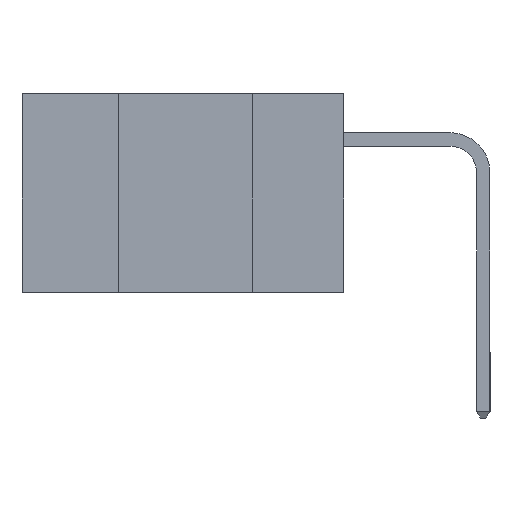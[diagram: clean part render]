
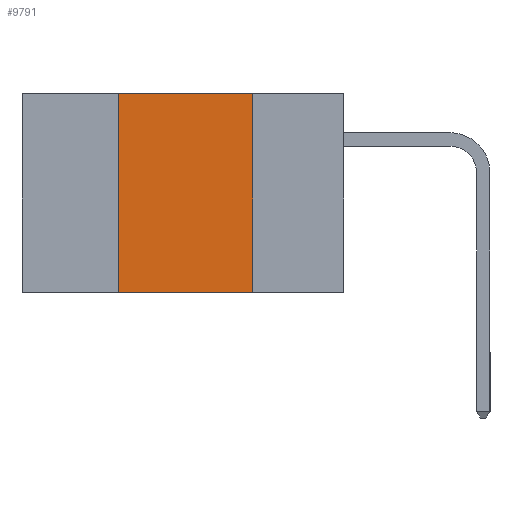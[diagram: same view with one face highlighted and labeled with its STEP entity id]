
A CAD part, left-side view. The second image highlights one B-rep face of the part: STEP entity #9791.
In plain terms, the highlighted planar face has unit normal (-1, 0, 0).
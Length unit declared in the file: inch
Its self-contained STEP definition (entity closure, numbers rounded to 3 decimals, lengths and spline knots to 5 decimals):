
#140 = VECTOR ( 'NONE', #741, 39.37008 ) ;
#741 = DIRECTION ( 'NONE',  ( 0., 0., 1. ) ) ;
#1108 = PLANE ( 'NONE',  #6056 ) ;
#1586 = LINE ( 'NONE', #14349, #6851 ) ;
#2267 = CARTESIAN_POINT ( 'NONE',  ( 0., 0.42, 0. ) ) ;
#2345 = DIRECTION ( 'NONE',  ( 0., -1., 0. ) ) ;
#3249 = CARTESIAN_POINT ( 'NONE',  ( 0., 0.17, -0.37 ) ) ;
#3289 = VERTEX_POINT ( 'NONE', #3249 ) ;
#3388 = VECTOR ( 'NONE', #4735, 39.37008 ) ;
#4735 = DIRECTION ( 'NONE',  ( 0., 0., -1. ) ) ;
#4743 = DIRECTION ( 'NONE',  ( 0., 0., -1. ) ) ;
#5548 = CARTESIAN_POINT ( 'NONE',  ( 0., 0.42, -0.37 ) ) ;
#5636 = ORIENTED_EDGE ( 'NONE', *, *, #16209, .T. ) ;
#6056 = AXIS2_PLACEMENT_3D ( 'NONE', #13560, #9617, #4743 ) ;
#6851 = VECTOR ( 'NONE', #9168, 39.37008 ) ;
#7109 = EDGE_CURVE ( 'NONE', #7541, #10866, #9341, .T. ) ;
#7370 = CARTESIAN_POINT ( 'NONE',  ( 0., 0.17, -0.37 ) ) ;
#7541 = VERTEX_POINT ( 'NONE', #13039 ) ;
#7627 = ORIENTED_EDGE ( 'NONE', *, *, #7109, .F. ) ;
#7679 = CARTESIAN_POINT ( 'NONE',  ( 0., 0.17, 0. ) ) ;
#9168 = DIRECTION ( 'NONE',  ( 0., -1., 0. ) ) ;
#9341 = LINE ( 'NONE', #5548, #140 ) ;
#9462 = VECTOR ( 'NONE', #2345, 39.37008 ) ;
#9617 = DIRECTION ( 'NONE',  ( 1., 0., 0. ) ) ;
#9791 = ADVANCED_FACE ( 'NONE', ( #11194 ), #1108, .F. ) ;
#9956 = CARTESIAN_POINT ( 'NONE',  ( 0., 0.6, 0. ) ) ;
#10866 = VERTEX_POINT ( 'NONE', #2267 ) ;
#10971 = EDGE_CURVE ( 'NONE', #11698, #3289, #13625, .T. ) ;
#11110 = ORIENTED_EDGE ( 'NONE', *, *, #10971, .F. ) ;
#11194 = FACE_OUTER_BOUND ( 'NONE', #11795, .T. ) ;
#11698 = VERTEX_POINT ( 'NONE', #7679 ) ;
#11795 = EDGE_LOOP ( 'NONE', ( #11110, #14088, #7627, #5636 ) ) ;
#13039 = CARTESIAN_POINT ( 'NONE',  ( 0., 0.42, -0.37 ) ) ;
#13560 = CARTESIAN_POINT ( 'NONE',  ( 0., 0.6, 0. ) ) ;
#13625 = LINE ( 'NONE', #7370, #3388 ) ;
#14088 = ORIENTED_EDGE ( 'NONE', *, *, #14184, .F. ) ;
#14184 = EDGE_CURVE ( 'NONE', #10866, #11698, #14870, .T. ) ;
#14349 = CARTESIAN_POINT ( 'NONE',  ( 0., 0.6, -0.37 ) ) ;
#14870 = LINE ( 'NONE', #9956, #9462 ) ;
#16209 = EDGE_CURVE ( 'NONE', #7541, #3289, #1586, .T. ) ;
